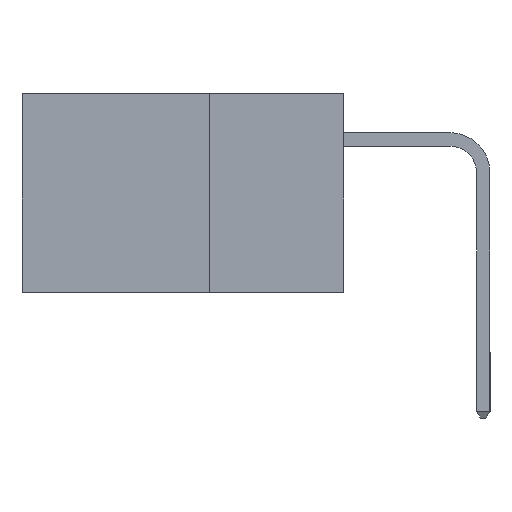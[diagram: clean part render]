
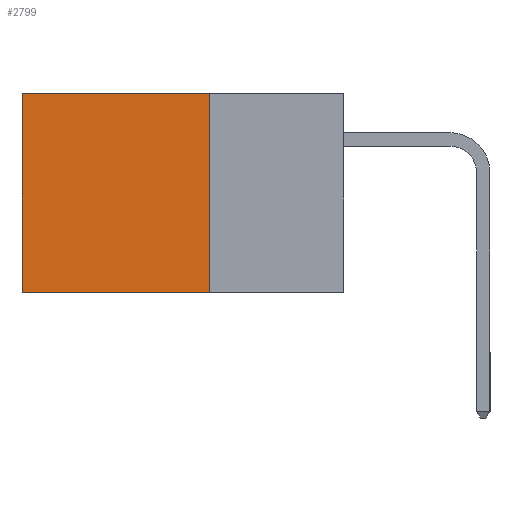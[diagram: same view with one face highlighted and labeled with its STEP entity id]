
A CAD part, left-side view. The second image highlights one B-rep face of the part: STEP entity #2799.
In plain terms, the highlighted planar face has unit normal (-1, 0, 0).
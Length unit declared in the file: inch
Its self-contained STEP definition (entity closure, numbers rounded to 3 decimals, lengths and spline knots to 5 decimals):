
#43 = VERTEX_POINT ( 'NONE', #3198 ) ;
#286 = FACE_OUTER_BOUND ( 'NONE', #9235, .T. ) ;
#1069 = VERTEX_POINT ( 'NONE', #9034 ) ;
#1257 = EDGE_CURVE ( 'NONE', #8257, #43, #6254, .T. ) ;
#1334 = EDGE_CURVE ( 'NONE', #6119, #1069, #7215, .T. ) ;
#1504 = CARTESIAN_POINT ( 'NONE',  ( 0.2615, 0.6, -0.37 ) ) ;
#1609 = VECTOR ( 'NONE', #7555, 39.37008 ) ;
#1771 = CARTESIAN_POINT ( 'NONE',  ( 0.2615, 0.25, -0.37 ) ) ;
#2482 = DIRECTION ( 'NONE',  ( 1., 0., 0. ) ) ;
#2584 = ORIENTED_EDGE ( 'NONE', *, *, #1257, .F. ) ;
#2799 = ADVANCED_FACE ( 'NONE', ( #286 ), #3209, .F. ) ;
#3119 = VECTOR ( 'NONE', #8756, 39.37008 ) ;
#3198 = CARTESIAN_POINT ( 'NONE',  ( 0.2615, 0.25, -0.37 ) ) ;
#3209 = PLANE ( 'NONE',  #6576 ) ;
#3429 = ORIENTED_EDGE ( 'NONE', *, *, #1334, .T. ) ;
#4048 = LINE ( 'NONE', #1771, #1609 ) ;
#4343 = DIRECTION ( 'NONE',  ( 0., 0., -1. ) ) ;
#4399 = CARTESIAN_POINT ( 'NONE',  ( 0.2615, 0.25, 0. ) ) ;
#4882 = CARTESIAN_POINT ( 'NONE',  ( 0.2615, 0.6, 0. ) ) ;
#5197 = ORIENTED_EDGE ( 'NONE', *, *, #8021, .F. ) ;
#5462 = ORIENTED_EDGE ( 'NONE', *, *, #8929, .T. ) ;
#5696 = DIRECTION ( 'NONE',  ( 0., 1., 0. ) ) ;
#6119 = VERTEX_POINT ( 'NONE', #4882 ) ;
#6184 = VECTOR ( 'NONE', #5696, 39.37008 ) ;
#6254 = LINE ( 'NONE', #9239, #7066 ) ;
#6576 = AXIS2_PLACEMENT_3D ( 'NONE', #8956, #2482, #8220 ) ;
#7066 = VECTOR ( 'NONE', #4343, 39.37008 ) ;
#7215 = LINE ( 'NONE', #1504, #3119 ) ;
#7555 = DIRECTION ( 'NONE',  ( 0., 1., 0. ) ) ;
#7804 = CARTESIAN_POINT ( 'NONE',  ( 0.2615, 0.25, 0. ) ) ;
#8021 = EDGE_CURVE ( 'NONE', #43, #1069, #4048, .T. ) ;
#8220 = DIRECTION ( 'NONE',  ( 0., 0., -1. ) ) ;
#8257 = VERTEX_POINT ( 'NONE', #4399 ) ;
#8756 = DIRECTION ( 'NONE',  ( 0., 0., -1. ) ) ;
#8929 = EDGE_CURVE ( 'NONE', #8257, #6119, #9255, .T. ) ;
#8956 = CARTESIAN_POINT ( 'NONE',  ( 0.2615, 0.25, -0.37 ) ) ;
#9034 = CARTESIAN_POINT ( 'NONE',  ( 0.2615, 0.6, -0.37 ) ) ;
#9235 = EDGE_LOOP ( 'NONE', ( #3429, #5197, #2584, #5462 ) ) ;
#9239 = CARTESIAN_POINT ( 'NONE',  ( 0.2615, 0.25, -0.37 ) ) ;
#9255 = LINE ( 'NONE', #7804, #6184 ) ;
